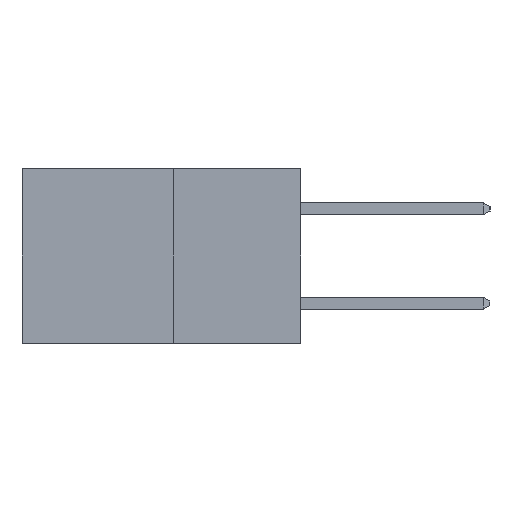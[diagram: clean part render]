
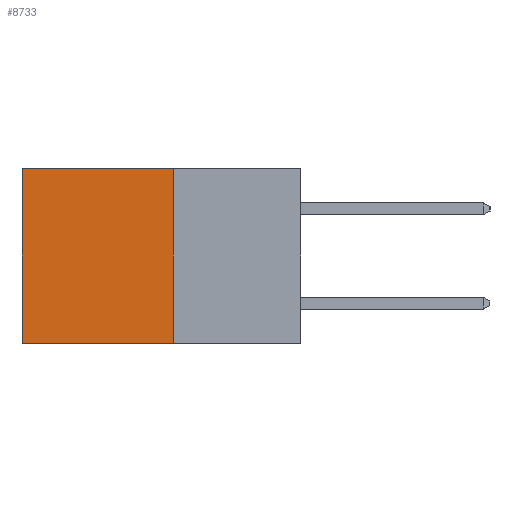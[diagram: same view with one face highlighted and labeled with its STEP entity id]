
A CAD part, left-side view. The second image highlights one B-rep face of the part: STEP entity #8733.
In plain terms, the highlighted planar face has unit normal (-1, 0, 0).
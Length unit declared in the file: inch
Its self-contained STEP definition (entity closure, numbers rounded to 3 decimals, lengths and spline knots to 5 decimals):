
#1095 = DIRECTION ( 'NONE',  ( 0., 0., -1. ) ) ;
#1337 = EDGE_LOOP ( 'NONE', ( #1843, #6079, #1924, #7476 ) ) ;
#1509 = CARTESIAN_POINT ( 'NONE',  ( 0.277, 0.27, 0. ) ) ;
#1843 = ORIENTED_EDGE ( 'NONE', *, *, #2576, .T. ) ;
#1888 = CARTESIAN_POINT ( 'NONE',  ( 0.277, 0.59, -0.37 ) ) ;
#1924 = ORIENTED_EDGE ( 'NONE', *, *, #15001, .F. ) ;
#2576 = EDGE_CURVE ( 'NONE', #16442, #16984, #13201, .T. ) ;
#2758 = CARTESIAN_POINT ( 'NONE',  ( 0.277, 0.27, -0.37 ) ) ;
#5031 = LINE ( 'NONE', #15995, #8958 ) ;
#5120 = CARTESIAN_POINT ( 'NONE',  ( 0.277, 0.27, -0.37 ) ) ;
#5372 = CARTESIAN_POINT ( 'NONE',  ( 0.277, 0.27, 0. ) ) ;
#5699 = VECTOR ( 'NONE', #14129, 39.37008 ) ;
#5730 = DIRECTION ( 'NONE',  ( 1., 0., 0. ) ) ;
#5859 = DIRECTION ( 'NONE',  ( 0., 1., 0. ) ) ;
#6079 = ORIENTED_EDGE ( 'NONE', *, *, #18163, .F. ) ;
#7264 = VERTEX_POINT ( 'NONE', #11552 ) ;
#7476 = ORIENTED_EDGE ( 'NONE', *, *, #9992, .T. ) ;
#8733 = ADVANCED_FACE ( 'NONE', ( #16149 ), #14411, .F. ) ;
#8958 = VECTOR ( 'NONE', #5859, 39.37008 ) ;
#9249 = AXIS2_PLACEMENT_3D ( 'NONE', #2758, #5730, #15869 ) ;
#9992 = EDGE_CURVE ( 'NONE', #14739, #16442, #17302, .T. ) ;
#11340 = CARTESIAN_POINT ( 'NONE',  ( 0.277, 0.59, 0. ) ) ;
#11552 = CARTESIAN_POINT ( 'NONE',  ( 0.277, 0.27, -0.37 ) ) ;
#13201 = LINE ( 'NONE', #1888, #17099 ) ;
#13806 = DIRECTION ( 'NONE',  ( 0., 0., -1. ) ) ;
#13941 = CARTESIAN_POINT ( 'NONE',  ( 0.277, 0.59, -0.37 ) ) ;
#14129 = DIRECTION ( 'NONE',  ( 0., 1., 0. ) ) ;
#14411 = PLANE ( 'NONE',  #9249 ) ;
#14739 = VERTEX_POINT ( 'NONE', #1509 ) ;
#14889 = VECTOR ( 'NONE', #13806, 39.37008 ) ;
#15001 = EDGE_CURVE ( 'NONE', #14739, #7264, #18765, .T. ) ;
#15869 = DIRECTION ( 'NONE',  ( 0., 0., -1. ) ) ;
#15995 = CARTESIAN_POINT ( 'NONE',  ( 0.277, 0.27, -0.37 ) ) ;
#16149 = FACE_OUTER_BOUND ( 'NONE', #1337, .T. ) ;
#16442 = VERTEX_POINT ( 'NONE', #11340 ) ;
#16984 = VERTEX_POINT ( 'NONE', #13941 ) ;
#17099 = VECTOR ( 'NONE', #1095, 39.37008 ) ;
#17302 = LINE ( 'NONE', #5372, #5699 ) ;
#18163 = EDGE_CURVE ( 'NONE', #7264, #16984, #5031, .T. ) ;
#18765 = LINE ( 'NONE', #5120, #14889 ) ;
